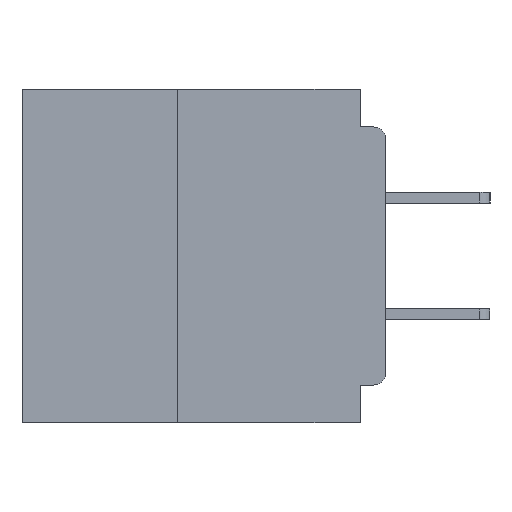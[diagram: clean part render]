
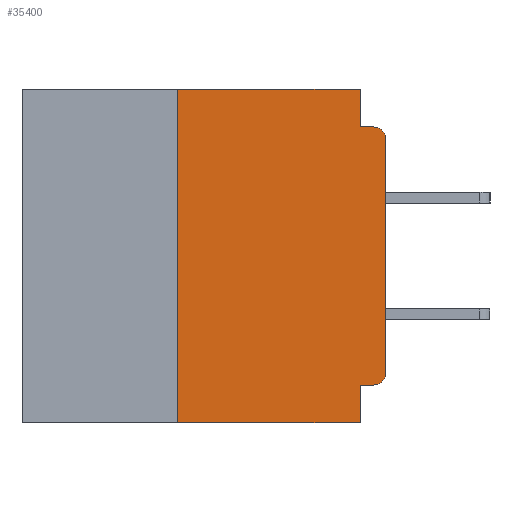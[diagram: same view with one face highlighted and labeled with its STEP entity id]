
A CAD part, left-side view. The second image highlights one B-rep face of the part: STEP entity #35400.
In plain terms, the highlighted planar face has unit normal (-1, 0, 0).
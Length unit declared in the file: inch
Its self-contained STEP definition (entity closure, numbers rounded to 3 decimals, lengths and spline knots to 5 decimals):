
#882 = VECTOR ( 'NONE', #5143, 39.37008 ) ;
#1574 = LINE ( 'NONE', #34565, #5065 ) ;
#2128 = EDGE_CURVE ( 'NONE', #6688, #46474, #39565, .T. ) ;
#3228 = AXIS2_PLACEMENT_3D ( 'NONE', #40836, #40486, #40478 ) ;
#3391 = FACE_OUTER_BOUND ( 'NONE', #21217, .T. ) ;
#3678 = ORIENTED_EDGE ( 'NONE', *, *, #37025, .T. ) ;
#4184 = CARTESIAN_POINT ( 'NONE',  ( 0., 0.031, -0.4 ) ) ;
#5065 = VECTOR ( 'NONE', #9339, 39.37008 ) ;
#5143 = DIRECTION ( 'NONE',  ( 0., -1., 0. ) ) ;
#5272 = VECTOR ( 'NONE', #31336, 39.37008 ) ;
#5768 = AXIS2_PLACEMENT_3D ( 'NONE', #11199, #36396, #14816 ) ;
#6073 = CARTESIAN_POINT ( 'NONE',  ( 0., 0.437, -0.4 ) ) ;
#6688 = VERTEX_POINT ( 'NONE', #20359 ) ;
#6951 = EDGE_CURVE ( 'NONE', #25608, #27649, #18110, .T. ) ;
#6966 = CARTESIAN_POINT ( 'NONE',  ( 0., 0.031, -0.045 ) ) ;
#7038 = VERTEX_POINT ( 'NONE', #19051 ) ;
#7554 = ORIENTED_EDGE ( 'NONE', *, *, #18618, .F. ) ;
#7790 = DIRECTION ( 'NONE',  ( 0., 0., -1. ) ) ;
#8132 = ORIENTED_EDGE ( 'NONE', *, *, #6951, .T. ) ;
#8255 = CARTESIAN_POINT ( 'NONE',  ( 0., 0.031, -0.4 ) ) ;
#9339 = DIRECTION ( 'NONE',  ( 0., 0., 1. ) ) ;
#9502 = VECTOR ( 'NONE', #23682, 39.37008 ) ;
#9948 = LINE ( 'NONE', #34933, #39754 ) ;
#11199 = CARTESIAN_POINT ( 'NONE',  ( 0., 0.015, -0.06 ) ) ;
#12339 = EDGE_CURVE ( 'NONE', #36640, #25075, #44544, .T. ) ;
#13358 = DIRECTION ( 'NONE',  ( 0., 1., 0. ) ) ;
#14452 = AXIS2_PLACEMENT_3D ( 'NONE', #15636, #40758, #19284 ) ;
#14816 = DIRECTION ( 'NONE',  ( 0., 0., -1. ) ) ;
#15636 = CARTESIAN_POINT ( 'NONE',  ( 0., 0.437, 0. ) ) ;
#16286 = CARTESIAN_POINT ( 'NONE',  ( 0., 0.031, 0. ) ) ;
#16382 = CARTESIAN_POINT ( 'NONE',  ( 0., 0., 0. ) ) ;
#17346 = VECTOR ( 'NONE', #44945, 39.37008 ) ;
#17833 = CARTESIAN_POINT ( 'NONE',  ( 0., 0.25, -0.4 ) ) ;
#18081 = VECTOR ( 'NONE', #7790, 39.37008 ) ;
#18110 = CIRCLE ( 'NONE', #5768, 0.015 ) ;
#18355 = ORIENTED_EDGE ( 'NONE', *, *, #29658, .F. ) ;
#18395 = ORIENTED_EDGE ( 'NONE', *, *, #32124, .F. ) ;
#18618 = EDGE_CURVE ( 'NONE', #23768, #25075, #26607, .T. ) ;
#19051 = CARTESIAN_POINT ( 'NONE',  ( 0., 0.25, 0. ) ) ;
#19090 = LINE ( 'NONE', #16382, #9502 ) ;
#19110 = VERTEX_POINT ( 'NONE', #6966 ) ;
#19126 = PLANE ( 'NONE',  #14452 ) ;
#19284 = DIRECTION ( 'NONE',  ( 0., 0., -1. ) ) ;
#19635 = LINE ( 'NONE', #16286, #17346 ) ;
#20359 = CARTESIAN_POINT ( 'NONE',  ( 0., 0.015, -0.355 ) ) ;
#20611 = CARTESIAN_POINT ( 'NONE',  ( 0., 0.437, 0. ) ) ;
#21217 = EDGE_LOOP ( 'NONE', ( #3678, #8132, #18395, #18355, #42124, #40383, #44148, #7554, #39926, #26823 ) ) ;
#23682 = DIRECTION ( 'NONE',  ( 0., 0., 1. ) ) ;
#23768 = VERTEX_POINT ( 'NONE', #37269 ) ;
#23977 = EDGE_CURVE ( 'NONE', #7038, #34410, #39251, .T. ) ;
#24142 = CARTESIAN_POINT ( 'NONE',  ( 0., 0.031, 0. ) ) ;
#24686 = EDGE_CURVE ( 'NONE', #6688, #23768, #9948, .T. ) ;
#25075 = VERTEX_POINT ( 'NONE', #8255 ) ;
#25608 = VERTEX_POINT ( 'NONE', #43343 ) ;
#26607 = LINE ( 'NONE', #4184, #18081 ) ;
#26782 = CARTESIAN_POINT ( 'NONE',  ( 0., 0., -0.045 ) ) ;
#26823 = ORIENTED_EDGE ( 'NONE', *, *, #2128, .T. ) ;
#27649 = VERTEX_POINT ( 'NONE', #36918 ) ;
#27891 = DIRECTION ( 'NONE',  ( 0., -1., 0. ) ) ;
#28575 = LINE ( 'NONE', #26782, #882 ) ;
#29658 = EDGE_CURVE ( 'NONE', #34410, #19110, #19635, .T. ) ;
#29816 = VECTOR ( 'NONE', #27891, 39.37008 ) ;
#31336 = DIRECTION ( 'NONE',  ( 0., -1., 0. ) ) ;
#32124 = EDGE_CURVE ( 'NONE', #19110, #27649, #28575, .T. ) ;
#34326 = CARTESIAN_POINT ( 'NONE',  ( 0., 0., -0.34 ) ) ;
#34410 = VERTEX_POINT ( 'NONE', #24142 ) ;
#34565 = CARTESIAN_POINT ( 'NONE',  ( 0., 0.25, -0.4 ) ) ;
#34933 = CARTESIAN_POINT ( 'NONE',  ( 0., 0., -0.355 ) ) ;
#35400 = ADVANCED_FACE ( 'NONE', ( #3391 ), #19126, .F. ) ;
#35609 = EDGE_CURVE ( 'NONE', #36640, #7038, #1574, .T. ) ;
#36396 = DIRECTION ( 'NONE',  ( -1., 0., 0. ) ) ;
#36640 = VERTEX_POINT ( 'NONE', #17833 ) ;
#36918 = CARTESIAN_POINT ( 'NONE',  ( 0., 0.015, -0.045 ) ) ;
#37025 = EDGE_CURVE ( 'NONE', #46474, #25608, #19090, .T. ) ;
#37269 = CARTESIAN_POINT ( 'NONE',  ( 0., 0.031, -0.355 ) ) ;
#39251 = LINE ( 'NONE', #20611, #29816 ) ;
#39565 = CIRCLE ( 'NONE', #3228, 0.015 ) ;
#39754 = VECTOR ( 'NONE', #13358, 39.37008 ) ;
#39926 = ORIENTED_EDGE ( 'NONE', *, *, #24686, .F. ) ;
#40383 = ORIENTED_EDGE ( 'NONE', *, *, #35609, .F. ) ;
#40478 = DIRECTION ( 'NONE',  ( 0., 0., -1. ) ) ;
#40486 = DIRECTION ( 'NONE',  ( -1., 0., 0. ) ) ;
#40758 = DIRECTION ( 'NONE',  ( 1., 0., 0. ) ) ;
#40836 = CARTESIAN_POINT ( 'NONE',  ( 0., 0.015, -0.34 ) ) ;
#42124 = ORIENTED_EDGE ( 'NONE', *, *, #23977, .F. ) ;
#43343 = CARTESIAN_POINT ( 'NONE',  ( 0., 0., -0.06 ) ) ;
#44148 = ORIENTED_EDGE ( 'NONE', *, *, #12339, .T. ) ;
#44544 = LINE ( 'NONE', #6073, #5272 ) ;
#44945 = DIRECTION ( 'NONE',  ( 0., 0., -1. ) ) ;
#46474 = VERTEX_POINT ( 'NONE', #34326 ) ;
